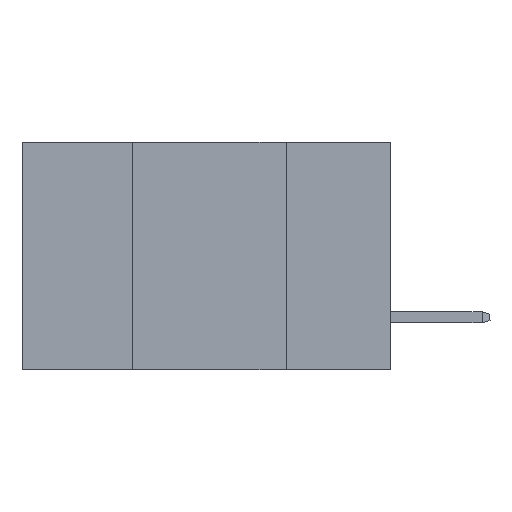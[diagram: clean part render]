
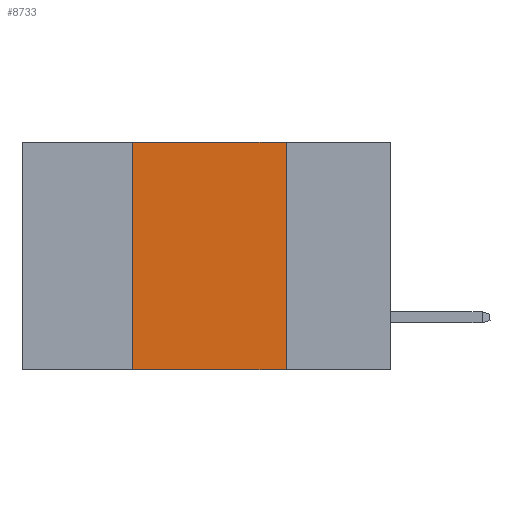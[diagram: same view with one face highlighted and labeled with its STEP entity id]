
A CAD part, left-side view. The second image highlights one B-rep face of the part: STEP entity #8733.
In plain terms, the highlighted planar face has unit normal (-1, 0, 0).
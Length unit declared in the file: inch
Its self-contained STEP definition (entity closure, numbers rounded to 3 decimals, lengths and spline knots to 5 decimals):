
#42 = ORIENTED_EDGE ( 'NONE', *, *, #12545, .F. ) ;
#242 = VERTEX_POINT ( 'NONE', #9481 ) ;
#444 = CARTESIAN_POINT ( 'NONE',  ( 0., 0.42, -0.37 ) ) ;
#761 = EDGE_LOOP ( 'NONE', ( #6858, #2200, #42, #3807 ) ) ;
#1247 = DIRECTION ( 'NONE',  ( 0., -1., 0. ) ) ;
#2200 = ORIENTED_EDGE ( 'NONE', *, *, #11148, .F. ) ;
#3479 = DIRECTION ( 'NONE',  ( 1., 0., 0. ) ) ;
#3807 = ORIENTED_EDGE ( 'NONE', *, *, #7868, .T. ) ;
#4160 = AXIS2_PLACEMENT_3D ( 'NONE', #12023, #3479, #10204 ) ;
#4546 = FACE_OUTER_BOUND ( 'NONE', #761, .T. ) ;
#4874 = VECTOR ( 'NONE', #12624, 39.37008 ) ;
#4930 = CARTESIAN_POINT ( 'NONE',  ( 0., 0.17, 0. ) ) ;
#6214 = VERTEX_POINT ( 'NONE', #10783 ) ;
#6269 = LINE ( 'NONE', #4930, #6565 ) ;
#6565 = VECTOR ( 'NONE', #11526, 39.37008 ) ;
#6858 = ORIENTED_EDGE ( 'NONE', *, *, #7093, .F. ) ;
#7055 = CARTESIAN_POINT ( 'NONE',  ( 0., 0.6, -0.37 ) ) ;
#7060 = LINE ( 'NONE', #7246, #11746 ) ;
#7093 = EDGE_CURVE ( 'NONE', #242, #6214, #6269, .T. ) ;
#7246 = CARTESIAN_POINT ( 'NONE',  ( 0., 0.6, 0. ) ) ;
#7868 = EDGE_CURVE ( 'NONE', #12508, #6214, #11808, .T. ) ;
#8431 = CARTESIAN_POINT ( 'NONE',  ( 0., 0.42, 0. ) ) ;
#8733 = ADVANCED_FACE ( 'NONE', ( #4546 ), #9263, .F. ) ;
#9263 = PLANE ( 'NONE',  #4160 ) ;
#9388 = CARTESIAN_POINT ( 'NONE',  ( 0., 0.42, 0. ) ) ;
#9481 = CARTESIAN_POINT ( 'NONE',  ( 0., 0.17, 0. ) ) ;
#9916 = VECTOR ( 'NONE', #11247, 39.37008 ) ;
#10204 = DIRECTION ( 'NONE',  ( 0., 0., -1. ) ) ;
#10219 = LINE ( 'NONE', #8431, #9916 ) ;
#10783 = CARTESIAN_POINT ( 'NONE',  ( 0., 0.17, -0.37 ) ) ;
#11148 = EDGE_CURVE ( 'NONE', #12538, #242, #7060, .T. ) ;
#11247 = DIRECTION ( 'NONE',  ( 0., 0., 1. ) ) ;
#11526 = DIRECTION ( 'NONE',  ( 0., 0., -1. ) ) ;
#11746 = VECTOR ( 'NONE', #1247, 39.37008 ) ;
#11808 = LINE ( 'NONE', #7055, #4874 ) ;
#12023 = CARTESIAN_POINT ( 'NONE',  ( 0., 0.6, 0. ) ) ;
#12508 = VERTEX_POINT ( 'NONE', #444 ) ;
#12538 = VERTEX_POINT ( 'NONE', #9388 ) ;
#12545 = EDGE_CURVE ( 'NONE', #12508, #12538, #10219, .T. ) ;
#12624 = DIRECTION ( 'NONE',  ( 0., -1., 0. ) ) ;
